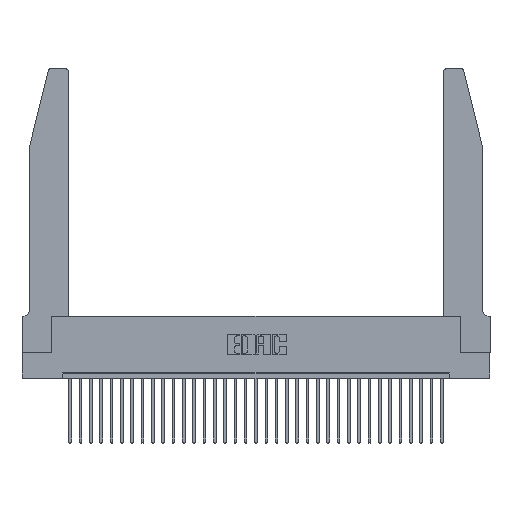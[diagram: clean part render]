
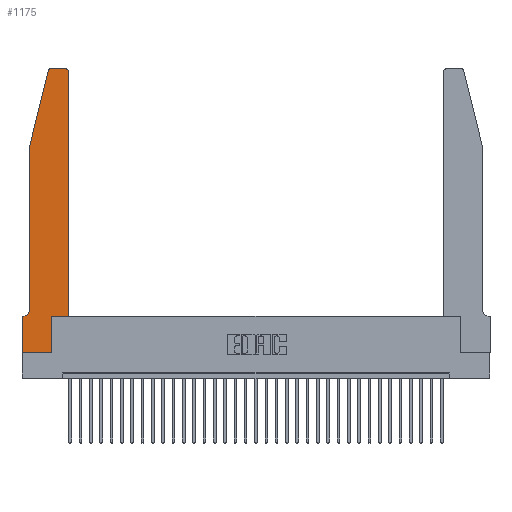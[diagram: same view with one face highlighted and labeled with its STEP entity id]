
A CAD part, top view. The second image highlights one B-rep face of the part: STEP entity #1175.
In plain terms, the highlighted planar face has unit normal (0, 0, 1).
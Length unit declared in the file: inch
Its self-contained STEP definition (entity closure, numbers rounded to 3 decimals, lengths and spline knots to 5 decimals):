
#282 = EDGE_CURVE ( 'NONE', #16507, #24529, #19548, .T. ) ;
#494 = DIRECTION ( 'NONE',  ( 1., 0., 0. ) ) ;
#1175 = ADVANCED_FACE ( 'NONE', ( #1792 ), #12080, .T. ) ;
#1792 = FACE_OUTER_BOUND ( 'NONE', #30989, .T. ) ;
#1795 = CARTESIAN_POINT ( 'NONE',  ( 0.2865, 0.35, 0.37 ) ) ;
#2861 = ORIENTED_EDGE ( 'NONE', *, *, #30061, .T. ) ;
#2893 = AXIS2_PLACEMENT_3D ( 'NONE', #19461, #4161, #11420 ) ;
#2932 = AXIS2_PLACEMENT_3D ( 'NONE', #14366, #11674, #24172 ) ;
#2953 = ORIENTED_EDGE ( 'NONE', *, *, #25470, .T. ) ;
#3016 = VECTOR ( 'NONE', #32975, 39.37008 ) ;
#3198 = CARTESIAN_POINT ( 'NONE',  ( 0.0755, 2., 0.37 ) ) ;
#3703 = LINE ( 'NONE', #12624, #19409 ) ;
#3727 = LINE ( 'NONE', #21597, #20644 ) ;
#4161 = DIRECTION ( 'NONE',  ( 0., 0., 1. ) ) ;
#4355 = VECTOR ( 'NONE', #23491, 39.37008 ) ;
#4955 = ORIENTED_EDGE ( 'NONE', *, *, #10032, .T. ) ;
#5206 = AXIS2_PLACEMENT_3D ( 'NONE', #15132, #25060, #9515 ) ;
#5765 = VERTEX_POINT ( 'NONE', #23183 ) ;
#6207 = EDGE_CURVE ( 'NONE', #20942, #26468, #14347, .T. ) ;
#6269 = CARTESIAN_POINT ( 'NONE',  ( 0.284, 2.75, 0.37 ) ) ;
#6529 = EDGE_CURVE ( 'NONE', #22775, #17918, #9102, .T. ) ;
#7452 = LINE ( 'NONE', #9618, #3016 ) ;
#7546 = VECTOR ( 'NONE', #494, 39.37008 ) ;
#7612 = CARTESIAN_POINT ( 'NONE',  ( 0., 0., 0.37 ) ) ;
#8580 = EDGE_CURVE ( 'NONE', #24425, #22102, #13806, .T. ) ;
#8637 = CARTESIAN_POINT ( 'NONE',  ( 0.284, 2.72, 0.37 ) ) ;
#9102 = LINE ( 'NONE', #26094, #33188 ) ;
#9515 = DIRECTION ( 'NONE',  ( 1., 0., 0. ) ) ;
#9618 = CARTESIAN_POINT ( 'NONE',  ( 0.0755, 2., 0.37 ) ) ;
#9954 = CARTESIAN_POINT ( 'NONE',  ( 0., 0., 0.37 ) ) ;
#10032 = EDGE_CURVE ( 'NONE', #26468, #30431, #3703, .T. ) ;
#10265 = LINE ( 'NONE', #3198, #23152 ) ;
#10955 = CARTESIAN_POINT ( 'NONE',  ( 0.4205, 2.75, 0.37 ) ) ;
#11171 = ORIENTED_EDGE ( 'NONE', *, *, #282, .T. ) ;
#11229 = CARTESIAN_POINT ( 'NONE',  ( 0.4505, 2.72, 0.37 ) ) ;
#11268 = EDGE_CURVE ( 'NONE', #17918, #33123, #17328, .T. ) ;
#11420 = DIRECTION ( 'NONE',  ( 1., 0., 0. ) ) ;
#11456 = DIRECTION ( 'NONE',  ( 0., -1., 0. ) ) ;
#11674 = DIRECTION ( 'NONE',  ( 0., 0., -1. ) ) ;
#12035 = AXIS2_PLACEMENT_3D ( 'NONE', #8637, #29075, #26601 ) ;
#12080 = PLANE ( 'NONE',  #5206 ) ;
#12624 = CARTESIAN_POINT ( 'NONE',  ( 0.4505, 0.35, 0.37 ) ) ;
#12723 = ORIENTED_EDGE ( 'NONE', *, *, #28091, .T. ) ;
#13432 = CARTESIAN_POINT ( 'NONE',  ( 0.25487, 2.72718, 0.37 ) ) ;
#13806 = LINE ( 'NONE', #21651, #33119 ) ;
#13891 = EDGE_CURVE ( 'NONE', #24036, #5765, #10265, .T. ) ;
#14200 = CARTESIAN_POINT ( 'NONE',  ( 0.4505, 0.35, 0.37 ) ) ;
#14347 = LINE ( 'NONE', #17891, #7546 ) ;
#14366 = CARTESIAN_POINT ( 'NONE',  ( 0.0055, 0.42, 0.37 ) ) ;
#15001 = DIRECTION ( 'NONE',  ( -0.239, -0.971, 0. ) ) ;
#15132 = CARTESIAN_POINT ( 'NONE',  ( 0., 0.35, 0.37 ) ) ;
#15237 = DIRECTION ( 'NONE',  ( 0., 1., 0. ) ) ;
#15713 = ORIENTED_EDGE ( 'NONE', *, *, #8580, .T. ) ;
#15753 = ORIENTED_EDGE ( 'NONE', *, *, #11268, .T. ) ;
#16507 = VERTEX_POINT ( 'NONE', #31164 ) ;
#17328 = LINE ( 'NONE', #9954, #23734 ) ;
#17607 = LINE ( 'NONE', #20704, #4355 ) ;
#17891 = CARTESIAN_POINT ( 'NONE',  ( 0.4505, 0.35, 0.37 ) ) ;
#17918 = VERTEX_POINT ( 'NONE', #7612 ) ;
#19409 = VECTOR ( 'NONE', #15237, 39.37008 ) ;
#19461 = CARTESIAN_POINT ( 'NONE',  ( 0.4205, 2.72, 0.37 ) ) ;
#19548 = CIRCLE ( 'NONE', #2932, 0.07 ) ;
#20017 = ORIENTED_EDGE ( 'NONE', *, *, #25817, .T. ) ;
#20286 = ORIENTED_EDGE ( 'NONE', *, *, #13891, .T. ) ;
#20644 = VECTOR ( 'NONE', #29556, 39.37008 ) ;
#20704 = CARTESIAN_POINT ( 'NONE',  ( 0.0755, 0.35, 0.37 ) ) ;
#20710 = CIRCLE ( 'NONE', #12035, 0.03 ) ;
#20942 = VERTEX_POINT ( 'NONE', #1795 ) ;
#21597 = CARTESIAN_POINT ( 'NONE',  ( 0.2865, 0.35, 0.37 ) ) ;
#21651 = CARTESIAN_POINT ( 'NONE',  ( 0.2605, 2.75, 0.37 ) ) ;
#22078 = CARTESIAN_POINT ( 'NONE',  ( 0.2865, 0., 0.37 ) ) ;
#22102 = VERTEX_POINT ( 'NONE', #6269 ) ;
#22775 = VERTEX_POINT ( 'NONE', #26892 ) ;
#23152 = VECTOR ( 'NONE', #15001, 39.37008 ) ;
#23183 = CARTESIAN_POINT ( 'NONE',  ( 0.0755, 2., 0.37 ) ) ;
#23491 = DIRECTION ( 'NONE',  ( -1., 0., 0. ) ) ;
#23734 = VECTOR ( 'NONE', #25272, 39.37008 ) ;
#24036 = VERTEX_POINT ( 'NONE', #13432 ) ;
#24124 = DIRECTION ( 'NONE',  ( -1., 0., 0. ) ) ;
#24172 = DIRECTION ( 'NONE',  ( -1., 0., 0. ) ) ;
#24425 = VERTEX_POINT ( 'NONE', #10955 ) ;
#24512 = ORIENTED_EDGE ( 'NONE', *, *, #31102, .T. ) ;
#24529 = VERTEX_POINT ( 'NONE', #29598 ) ;
#24603 = ORIENTED_EDGE ( 'NONE', *, *, #6529, .T. ) ;
#25060 = DIRECTION ( 'NONE',  ( 0., 0., 1. ) ) ;
#25272 = DIRECTION ( 'NONE',  ( 1., 0., 0. ) ) ;
#25470 = EDGE_CURVE ( 'NONE', #24529, #22775, #17607, .T. ) ;
#25817 = EDGE_CURVE ( 'NONE', #30431, #24425, #32032, .T. ) ;
#26094 = CARTESIAN_POINT ( 'NONE',  ( 0., 0., 0.37 ) ) ;
#26468 = VERTEX_POINT ( 'NONE', #14200 ) ;
#26601 = DIRECTION ( 'NONE',  ( 1., 0., 0. ) ) ;
#26892 = CARTESIAN_POINT ( 'NONE',  ( 0., 0.35, 0.37 ) ) ;
#28091 = EDGE_CURVE ( 'NONE', #33123, #20942, #3727, .T. ) ;
#29075 = DIRECTION ( 'NONE',  ( 0., 0., 1. ) ) ;
#29556 = DIRECTION ( 'NONE',  ( 0., 1., 0. ) ) ;
#29598 = CARTESIAN_POINT ( 'NONE',  ( 0.0055, 0.35, 0.37 ) ) ;
#30061 = EDGE_CURVE ( 'NONE', #5765, #16507, #7452, .T. ) ;
#30431 = VERTEX_POINT ( 'NONE', #11229 ) ;
#30833 = ORIENTED_EDGE ( 'NONE', *, *, #6207, .T. ) ;
#30989 = EDGE_LOOP ( 'NONE', ( #15713, #24512, #20286, #2861, #11171, #2953, #24603, #15753, #12723, #30833, #4955, #20017 ) ) ;
#31102 = EDGE_CURVE ( 'NONE', #22102, #24036, #20710, .T. ) ;
#31164 = CARTESIAN_POINT ( 'NONE',  ( 0.0755, 0.42, 0.37 ) ) ;
#32032 = CIRCLE ( 'NONE', #2893, 0.03 ) ;
#32975 = DIRECTION ( 'NONE',  ( 0., -1., 0. ) ) ;
#33119 = VECTOR ( 'NONE', #24124, 39.37008 ) ;
#33123 = VERTEX_POINT ( 'NONE', #22078 ) ;
#33188 = VECTOR ( 'NONE', #11456, 39.37008 ) ;
